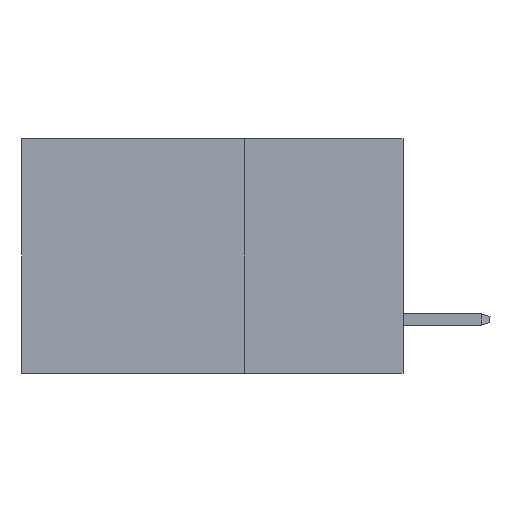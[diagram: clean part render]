
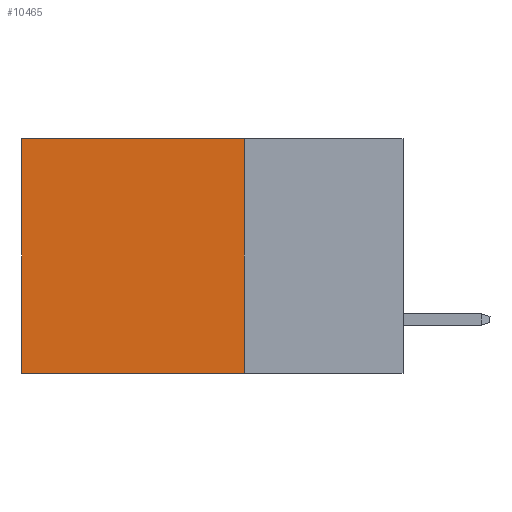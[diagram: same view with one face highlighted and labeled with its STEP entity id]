
A CAD part, left-side view. The second image highlights one B-rep face of the part: STEP entity #10465.
In plain terms, the highlighted planar face has unit normal (-1, 0, 0).
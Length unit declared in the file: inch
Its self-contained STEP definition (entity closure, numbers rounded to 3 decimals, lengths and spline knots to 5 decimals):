
#318 = ORIENTED_EDGE ( 'NONE', *, *, #1497, .T. ) ;
#546 = FACE_OUTER_BOUND ( 'NONE', #6306, .T. ) ;
#659 = CARTESIAN_POINT ( 'NONE',  ( 0.2875, 0.6, -0.37 ) ) ;
#704 = AXIS2_PLACEMENT_3D ( 'NONE', #1352, #2905, #3874 ) ;
#1352 = CARTESIAN_POINT ( 'NONE',  ( 0.2875, 0.25, 0. ) ) ;
#1481 = EDGE_CURVE ( 'NONE', #8515, #5613, #5776, .T. ) ;
#1497 = EDGE_CURVE ( 'NONE', #5613, #4433, #9363, .T. ) ;
#1910 = DIRECTION ( 'NONE',  ( 0., 1., 0. ) ) ;
#1962 = CARTESIAN_POINT ( 'NONE',  ( 0.2875, 0.6, 0. ) ) ;
#2186 = VECTOR ( 'NONE', #2403, 39.37008 ) ;
#2403 = DIRECTION ( 'NONE',  ( 0., 0., -1. ) ) ;
#2569 = LINE ( 'NONE', #9168, #2186 ) ;
#2905 = DIRECTION ( 'NONE',  ( 1., 0., 0. ) ) ;
#3107 = VECTOR ( 'NONE', #1910, 39.37008 ) ;
#3721 = PLANE ( 'NONE',  #704 ) ;
#3874 = DIRECTION ( 'NONE',  ( 0., 0., -1. ) ) ;
#4040 = VERTEX_POINT ( 'NONE', #6609 ) ;
#4143 = VECTOR ( 'NONE', #6817, 39.37008 ) ;
#4433 = VERTEX_POINT ( 'NONE', #659 ) ;
#5613 = VERTEX_POINT ( 'NONE', #8251 ) ;
#5776 = LINE ( 'NONE', #9949, #3107 ) ;
#6174 = ORIENTED_EDGE ( 'NONE', *, *, #6205, .F. ) ;
#6205 = EDGE_CURVE ( 'NONE', #8515, #4040, #2569, .T. ) ;
#6306 = EDGE_LOOP ( 'NONE', ( #318, #8837, #6174, #8668 ) ) ;
#6590 = LINE ( 'NONE', #8391, #8827 ) ;
#6609 = CARTESIAN_POINT ( 'NONE',  ( 0.2875, 0.25, -0.37 ) ) ;
#6817 = DIRECTION ( 'NONE',  ( 0., 0., -1. ) ) ;
#8017 = CARTESIAN_POINT ( 'NONE',  ( 0.2875, 0.25, 0. ) ) ;
#8251 = CARTESIAN_POINT ( 'NONE',  ( 0.2875, 0.6, 0. ) ) ;
#8391 = CARTESIAN_POINT ( 'NONE',  ( 0.2875, 0.25, -0.37 ) ) ;
#8515 = VERTEX_POINT ( 'NONE', #8017 ) ;
#8668 = ORIENTED_EDGE ( 'NONE', *, *, #1481, .T. ) ;
#8827 = VECTOR ( 'NONE', #9140, 39.37008 ) ;
#8837 = ORIENTED_EDGE ( 'NONE', *, *, #10237, .F. ) ;
#9140 = DIRECTION ( 'NONE',  ( 0., 1., 0. ) ) ;
#9168 = CARTESIAN_POINT ( 'NONE',  ( 0.2875, 0.25, 0. ) ) ;
#9363 = LINE ( 'NONE', #1962, #4143 ) ;
#9949 = CARTESIAN_POINT ( 'NONE',  ( 0.2875, 0.25, 0. ) ) ;
#10237 = EDGE_CURVE ( 'NONE', #4040, #4433, #6590, .T. ) ;
#10465 = ADVANCED_FACE ( 'NONE', ( #546 ), #3721, .F. ) ;
